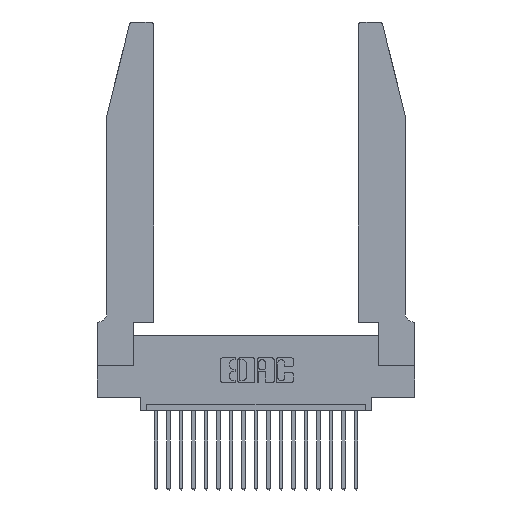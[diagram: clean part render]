
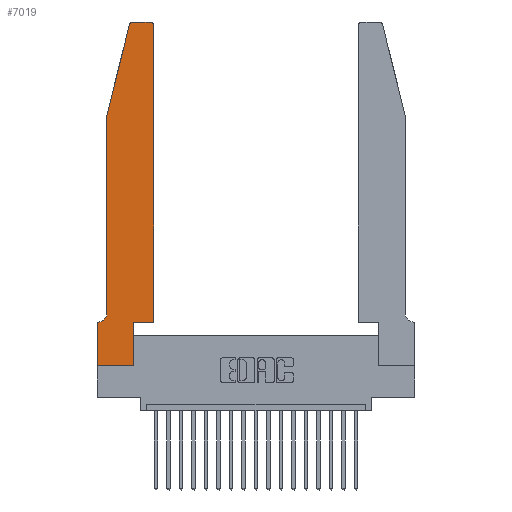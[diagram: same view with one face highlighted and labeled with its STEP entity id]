
A CAD part, top view. The second image highlights one B-rep face of the part: STEP entity #7019.
In plain terms, the highlighted planar face has unit normal (0, 0, 1).
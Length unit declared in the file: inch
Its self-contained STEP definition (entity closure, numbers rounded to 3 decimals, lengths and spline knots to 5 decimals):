
#406 = EDGE_CURVE ( 'NONE', #12239, #11815, #20265, .T. ) ;
#705 = CARTESIAN_POINT ( 'NONE',  ( 0.4505, 0.35, 0.37 ) ) ;
#741 = CARTESIAN_POINT ( 'NONE',  ( 0.0055, 0.35, 0.37 ) ) ;
#844 = FACE_OUTER_BOUND ( 'NONE', #5410, .T. ) ;
#984 = AXIS2_PLACEMENT_3D ( 'NONE', #5351, #16748, #13711 ) ;
#1707 = VECTOR ( 'NONE', #5614, 39.37008 ) ;
#1769 = DIRECTION ( 'NONE',  ( 0., -1., 0. ) ) ;
#2226 = DIRECTION ( 'NONE',  ( 1., 0., 0. ) ) ;
#2536 = ORIENTED_EDGE ( 'NONE', *, *, #13867, .T. ) ;
#2564 = VECTOR ( 'NONE', #2226, 39.37008 ) ;
#2792 = EDGE_CURVE ( 'NONE', #15010, #19532, #20894, .T. ) ;
#2922 = VERTEX_POINT ( 'NONE', #10705 ) ;
#3101 = ORIENTED_EDGE ( 'NONE', *, *, #14621, .T. ) ;
#3230 = ORIENTED_EDGE ( 'NONE', *, *, #18803, .T. ) ;
#3467 = CARTESIAN_POINT ( 'NONE',  ( 0., 0.35, 0.37 ) ) ;
#3762 = AXIS2_PLACEMENT_3D ( 'NONE', #16676, #6927, #18354 ) ;
#3844 = CIRCLE ( 'NONE', #5924, 0.07 ) ;
#3968 = CARTESIAN_POINT ( 'NONE',  ( 0.284, 2.75, 0.37 ) ) ;
#4132 = VERTEX_POINT ( 'NONE', #15618 ) ;
#4751 = DIRECTION ( 'NONE',  ( 0., 1., 0. ) ) ;
#4819 = CARTESIAN_POINT ( 'NONE',  ( 0.2605, 2.75, 0.37 ) ) ;
#5002 = VERTEX_POINT ( 'NONE', #9761 ) ;
#5351 = CARTESIAN_POINT ( 'NONE',  ( 0.4205, 2.72, 0.37 ) ) ;
#5410 = EDGE_LOOP ( 'NONE', ( #12043, #17725, #3230, #9411, #15786, #10906, #19510, #20650, #19558, #2536, #3101, #6246 ) ) ;
#5614 = DIRECTION ( 'NONE',  ( 1., 0., 0. ) ) ;
#5699 = EDGE_CURVE ( 'NONE', #14148, #5002, #12407, .T. ) ;
#5924 = AXIS2_PLACEMENT_3D ( 'NONE', #10465, #18653, #8968 ) ;
#6086 = VECTOR ( 'NONE', #1769, 39.37008 ) ;
#6246 = ORIENTED_EDGE ( 'NONE', *, *, #17227, .T. ) ;
#6600 = VERTEX_POINT ( 'NONE', #7163 ) ;
#6921 = CARTESIAN_POINT ( 'NONE',  ( 0.0755, 0.35, 0.37 ) ) ;
#6927 = DIRECTION ( 'NONE',  ( 0., 0., 1. ) ) ;
#7019 = ADVANCED_FACE ( 'NONE', ( #844 ), #8745, .T. ) ;
#7050 = LINE ( 'NONE', #14790, #15469 ) ;
#7163 = CARTESIAN_POINT ( 'NONE',  ( 0.4505, 0.35, 0.37 ) ) ;
#7395 = VECTOR ( 'NONE', #11234, 39.37008 ) ;
#7607 = LINE ( 'NONE', #705, #1707 ) ;
#7726 = CIRCLE ( 'NONE', #984, 0.03 ) ;
#8745 = PLANE ( 'NONE',  #3762 ) ;
#8910 = CARTESIAN_POINT ( 'NONE',  ( 0.0755, 2., 0.37 ) ) ;
#8968 = DIRECTION ( 'NONE',  ( -1., 0., 0. ) ) ;
#9065 = EDGE_CURVE ( 'NONE', #16490, #2922, #13814, .T. ) ;
#9411 = ORIENTED_EDGE ( 'NONE', *, *, #5699, .T. ) ;
#9761 = CARTESIAN_POINT ( 'NONE',  ( 0.0755, 0.42, 0.37 ) ) ;
#10029 = LINE ( 'NONE', #15922, #11059 ) ;
#10369 = EDGE_CURVE ( 'NONE', #17275, #12239, #15667, .T. ) ;
#10465 = CARTESIAN_POINT ( 'NONE',  ( 0.0055, 0.42, 0.37 ) ) ;
#10582 = CARTESIAN_POINT ( 'NONE',  ( 0.4205, 2.75, 0.37 ) ) ;
#10705 = CARTESIAN_POINT ( 'NONE',  ( 0.2865, 0., 0.37 ) ) ;
#10906 = ORIENTED_EDGE ( 'NONE', *, *, #2792, .T. ) ;
#11059 = VECTOR ( 'NONE', #4751, 39.37008 ) ;
#11145 = EDGE_CURVE ( 'NONE', #2922, #15946, #10029, .T. ) ;
#11165 = CARTESIAN_POINT ( 'NONE',  ( 0.0755, 2., 0.37 ) ) ;
#11234 = DIRECTION ( 'NONE',  ( -0.239, -0.971, 0. ) ) ;
#11576 = CARTESIAN_POINT ( 'NONE',  ( 0., 0., 0.37 ) ) ;
#11815 = VERTEX_POINT ( 'NONE', #18146 ) ;
#12043 = ORIENTED_EDGE ( 'NONE', *, *, #10369, .T. ) ;
#12239 = VERTEX_POINT ( 'NONE', #3968 ) ;
#12278 = CARTESIAN_POINT ( 'NONE',  ( 0.284, 2.72, 0.37 ) ) ;
#12407 = LINE ( 'NONE', #19304, #12673 ) ;
#12673 = VECTOR ( 'NONE', #19229, 39.37008 ) ;
#13139 = DIRECTION ( 'NONE',  ( -1., 0., 0. ) ) ;
#13287 = EDGE_CURVE ( 'NONE', #19532, #16490, #20346, .T. ) ;
#13563 = VECTOR ( 'NONE', #13139, 39.37008 ) ;
#13711 = DIRECTION ( 'NONE',  ( 1., 0., 0. ) ) ;
#13814 = LINE ( 'NONE', #20365, #2564 ) ;
#13867 = EDGE_CURVE ( 'NONE', #15946, #6600, #7607, .T. ) ;
#13955 = CARTESIAN_POINT ( 'NONE',  ( 0.2865, 0.35, 0.37 ) ) ;
#14148 = VERTEX_POINT ( 'NONE', #8910 ) ;
#14283 = DIRECTION ( 'NONE',  ( -1., 0., 0. ) ) ;
#14511 = CARTESIAN_POINT ( 'NONE',  ( 0., 0., 0.37 ) ) ;
#14621 = EDGE_CURVE ( 'NONE', #6600, #4132, #7050, .T. ) ;
#14790 = CARTESIAN_POINT ( 'NONE',  ( 0.4505, 0.35, 0.37 ) ) ;
#15010 = VERTEX_POINT ( 'NONE', #741 ) ;
#15469 = VECTOR ( 'NONE', #19395, 39.37008 ) ;
#15618 = CARTESIAN_POINT ( 'NONE',  ( 0.4505, 2.72, 0.37 ) ) ;
#15667 = LINE ( 'NONE', #4819, #18679 ) ;
#15786 = ORIENTED_EDGE ( 'NONE', *, *, #18468, .T. ) ;
#15799 = DIRECTION ( 'NONE',  ( 1., 0., 0. ) ) ;
#15922 = CARTESIAN_POINT ( 'NONE',  ( 0.2865, 0.35, 0.37 ) ) ;
#15946 = VERTEX_POINT ( 'NONE', #13955 ) ;
#16305 = LINE ( 'NONE', #11165, #7395 ) ;
#16490 = VERTEX_POINT ( 'NONE', #14511 ) ;
#16676 = CARTESIAN_POINT ( 'NONE',  ( 0., 0.35, 0.37 ) ) ;
#16748 = DIRECTION ( 'NONE',  ( 0., 0., 1. ) ) ;
#17227 = EDGE_CURVE ( 'NONE', #4132, #17275, #7726, .T. ) ;
#17275 = VERTEX_POINT ( 'NONE', #10582 ) ;
#17725 = ORIENTED_EDGE ( 'NONE', *, *, #406, .T. ) ;
#18146 = CARTESIAN_POINT ( 'NONE',  ( 0.25487, 2.72718, 0.37 ) ) ;
#18354 = DIRECTION ( 'NONE',  ( 1., 0., 0. ) ) ;
#18468 = EDGE_CURVE ( 'NONE', #5002, #15010, #3844, .T. ) ;
#18653 = DIRECTION ( 'NONE',  ( 0., 0., -1. ) ) ;
#18679 = VECTOR ( 'NONE', #14283, 39.37008 ) ;
#18803 = EDGE_CURVE ( 'NONE', #11815, #14148, #16305, .T. ) ;
#18977 = DIRECTION ( 'NONE',  ( 0., 0., 1. ) ) ;
#19106 = AXIS2_PLACEMENT_3D ( 'NONE', #12278, #18977, #15799 ) ;
#19229 = DIRECTION ( 'NONE',  ( 0., -1., 0. ) ) ;
#19304 = CARTESIAN_POINT ( 'NONE',  ( 0.0755, 2., 0.37 ) ) ;
#19395 = DIRECTION ( 'NONE',  ( 0., 1., 0. ) ) ;
#19510 = ORIENTED_EDGE ( 'NONE', *, *, #13287, .T. ) ;
#19532 = VERTEX_POINT ( 'NONE', #3467 ) ;
#19558 = ORIENTED_EDGE ( 'NONE', *, *, #11145, .T. ) ;
#20265 = CIRCLE ( 'NONE', #19106, 0.03 ) ;
#20346 = LINE ( 'NONE', #11576, #6086 ) ;
#20365 = CARTESIAN_POINT ( 'NONE',  ( 0., 0., 0.37 ) ) ;
#20650 = ORIENTED_EDGE ( 'NONE', *, *, #9065, .T. ) ;
#20894 = LINE ( 'NONE', #6921, #13563 ) ;
